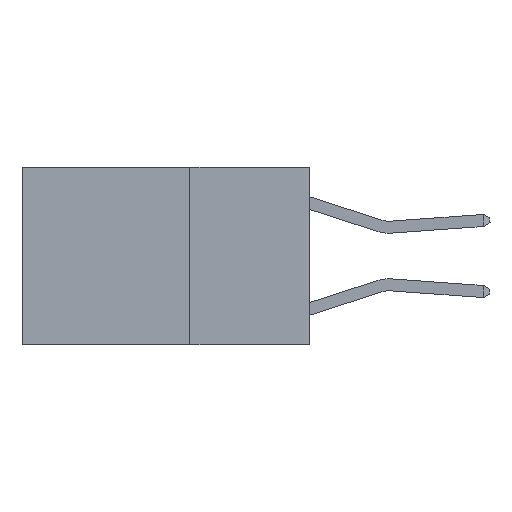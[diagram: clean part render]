
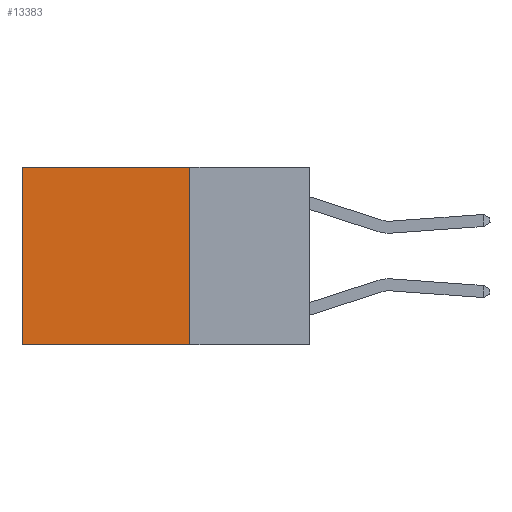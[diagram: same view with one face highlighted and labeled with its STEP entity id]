
A CAD part, left-side view. The second image highlights one B-rep face of the part: STEP entity #13383.
In plain terms, the highlighted planar face has unit normal (-1, 0, 0).
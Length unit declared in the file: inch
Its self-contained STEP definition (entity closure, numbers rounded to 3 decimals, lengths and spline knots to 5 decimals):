
#561 = DIRECTION ( 'NONE',  ( 0., 0., -1. ) ) ;
#749 = CARTESIAN_POINT ( 'NONE',  ( 0.2625, 0.25, -0.37 ) ) ;
#1915 = LINE ( 'NONE', #749, #14719 ) ;
#1974 = VECTOR ( 'NONE', #13381, 39.37008 ) ;
#3755 = CARTESIAN_POINT ( 'NONE',  ( 0.2625, 0.25, 0. ) ) ;
#3875 = CARTESIAN_POINT ( 'NONE',  ( 0.2625, 0.25, 0. ) ) ;
#3884 = EDGE_CURVE ( 'NONE', #15323, #9896, #5447, .T. ) ;
#4643 = CARTESIAN_POINT ( 'NONE',  ( 0.2625, 0.25, -0.37 ) ) ;
#4806 = VERTEX_POINT ( 'NONE', #13080 ) ;
#5447 = LINE ( 'NONE', #6136, #1974 ) ;
#5487 = ORIENTED_EDGE ( 'NONE', *, *, #5505, .T. ) ;
#5505 = EDGE_CURVE ( 'NONE', #4806, #15323, #11131, .T. ) ;
#5531 = LINE ( 'NONE', #8226, #9585 ) ;
#5763 = VERTEX_POINT ( 'NONE', #4643 ) ;
#5779 = EDGE_CURVE ( 'NONE', #5763, #9896, #1915, .T. ) ;
#6136 = CARTESIAN_POINT ( 'NONE',  ( 0.2625, 0.6, 0. ) ) ;
#7706 = DIRECTION ( 'NONE',  ( 1., 0., 0. ) ) ;
#7710 = EDGE_CURVE ( 'NONE', #4806, #5763, #5531, .T. ) ;
#7941 = VECTOR ( 'NONE', #11158, 39.37008 ) ;
#8022 = ORIENTED_EDGE ( 'NONE', *, *, #5779, .F. ) ;
#8226 = CARTESIAN_POINT ( 'NONE',  ( 0.2625, 0.25, 0. ) ) ;
#9585 = VECTOR ( 'NONE', #561, 39.37008 ) ;
#9896 = VERTEX_POINT ( 'NONE', #15266 ) ;
#10844 = ORIENTED_EDGE ( 'NONE', *, *, #3884, .T. ) ;
#11131 = LINE ( 'NONE', #3755, #7941 ) ;
#11158 = DIRECTION ( 'NONE',  ( 0., 1., 0. ) ) ;
#12158 = DIRECTION ( 'NONE',  ( 0., 0., -1. ) ) ;
#12913 = CARTESIAN_POINT ( 'NONE',  ( 0.2625, 0.6, 0. ) ) ;
#13080 = CARTESIAN_POINT ( 'NONE',  ( 0.2625, 0.25, 0. ) ) ;
#13253 = DIRECTION ( 'NONE',  ( 0., 1., 0. ) ) ;
#13381 = DIRECTION ( 'NONE',  ( 0., 0., -1. ) ) ;
#13383 = ADVANCED_FACE ( 'NONE', ( #14578 ), #14920, .F. ) ;
#13821 = EDGE_LOOP ( 'NONE', ( #10844, #8022, #14429, #5487 ) ) ;
#14258 = AXIS2_PLACEMENT_3D ( 'NONE', #3875, #7706, #12158 ) ;
#14429 = ORIENTED_EDGE ( 'NONE', *, *, #7710, .F. ) ;
#14578 = FACE_OUTER_BOUND ( 'NONE', #13821, .T. ) ;
#14719 = VECTOR ( 'NONE', #13253, 39.37008 ) ;
#14920 = PLANE ( 'NONE',  #14258 ) ;
#15266 = CARTESIAN_POINT ( 'NONE',  ( 0.2625, 0.6, -0.37 ) ) ;
#15323 = VERTEX_POINT ( 'NONE', #12913 ) ;
